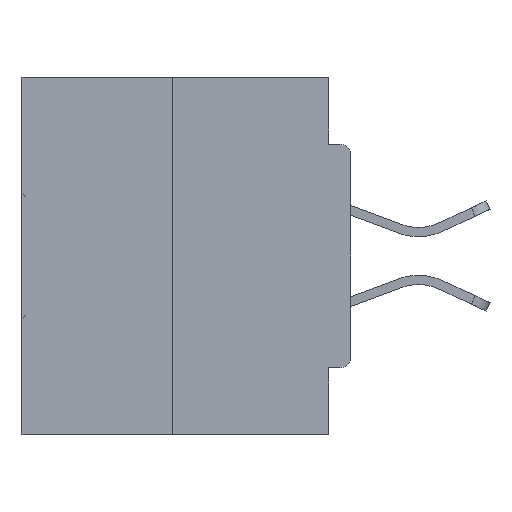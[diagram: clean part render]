
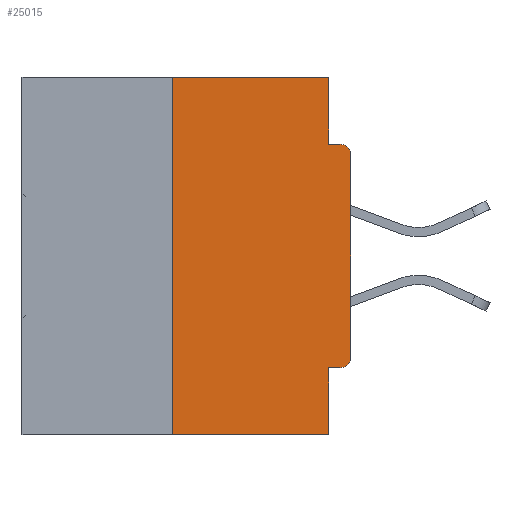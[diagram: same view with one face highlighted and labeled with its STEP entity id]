
A CAD part, left-side view. The second image highlights one B-rep face of the part: STEP entity #25015.
In plain terms, the highlighted planar face has unit normal (-1, 0, 0).
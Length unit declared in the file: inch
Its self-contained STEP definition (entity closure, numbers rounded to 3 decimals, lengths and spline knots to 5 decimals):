
#209 = VERTEX_POINT ( 'NONE', #27853 ) ;
#298 = CARTESIAN_POINT ( 'NONE',  ( 0., 0.25, 0. ) ) ;
#849 = ORIENTED_EDGE ( 'NONE', *, *, #33226, .T. ) ;
#915 = VECTOR ( 'NONE', #22588, 39.37008 ) ;
#1058 = LINE ( 'NONE', #39771, #12234 ) ;
#1157 = DIRECTION ( 'NONE',  ( 0., 0., -1. ) ) ;
#1381 = CARTESIAN_POINT ( 'NONE',  ( 0., 0., -0.4065 ) ) ;
#1384 = VERTEX_POINT ( 'NONE', #38906 ) ;
#1772 = ORIENTED_EDGE ( 'NONE', *, *, #12917, .T. ) ;
#2313 = CARTESIAN_POINT ( 'NONE',  ( 0., 0.031, -0.5 ) ) ;
#2521 = ORIENTED_EDGE ( 'NONE', *, *, #5078, .T. ) ;
#3207 = CARTESIAN_POINT ( 'NONE',  ( 0., 0.031, -0.4065 ) ) ;
#3614 = EDGE_CURVE ( 'NONE', #1384, #21017, #34693, .T. ) ;
#3821 = LINE ( 'NONE', #11021, #28789 ) ;
#3996 = VERTEX_POINT ( 'NONE', #16469 ) ;
#5057 = ORIENTED_EDGE ( 'NONE', *, *, #3614, .F. ) ;
#5078 = EDGE_CURVE ( 'NONE', #3996, #27350, #22658, .T. ) ;
#5991 = EDGE_CURVE ( 'NONE', #209, #16376, #36353, .T. ) ;
#6490 = CARTESIAN_POINT ( 'NONE',  ( 0., 0.25, 0. ) ) ;
#6495 = LINE ( 'NONE', #22873, #915 ) ;
#8624 = EDGE_CURVE ( 'NONE', #27197, #25356, #6495, .T. ) ;
#9118 = CARTESIAN_POINT ( 'NONE',  ( 0., 0.015, -0.3915 ) ) ;
#9577 = CARTESIAN_POINT ( 'NONE',  ( 0., 0., 0. ) ) ;
#10607 = VERTEX_POINT ( 'NONE', #32449 ) ;
#10872 = CARTESIAN_POINT ( 'NONE',  ( 0., 0.031, -0.5 ) ) ;
#11021 = CARTESIAN_POINT ( 'NONE',  ( 0., 0.46, -0.5 ) ) ;
#11678 = EDGE_LOOP ( 'NONE', ( #41995, #12970, #14958, #31051, #5057, #1772, #2521, #849, #37008, #13912 ) ) ;
#11947 = DIRECTION ( 'NONE',  ( 0., -1., 0. ) ) ;
#12234 = VECTOR ( 'NONE', #40074, 39.37008 ) ;
#12376 = DIRECTION ( 'NONE',  ( 0., 0., -1. ) ) ;
#12406 = DIRECTION ( 'NONE',  ( 0., 0., 1. ) ) ;
#12452 = VECTOR ( 'NONE', #11947, 39.37008 ) ;
#12458 = EDGE_CURVE ( 'NONE', #25356, #10607, #29871, .T. ) ;
#12851 = VERTEX_POINT ( 'NONE', #10872 ) ;
#12860 = EDGE_CURVE ( 'NONE', #209, #12851, #3821, .T. ) ;
#12917 = EDGE_CURVE ( 'NONE', #1384, #3996, #36448, .T. ) ;
#12970 = ORIENTED_EDGE ( 'NONE', *, *, #5991, .F. ) ;
#13542 = LINE ( 'NONE', #2313, #17114 ) ;
#13912 = ORIENTED_EDGE ( 'NONE', *, *, #8624, .F. ) ;
#14000 = DIRECTION ( 'NONE',  ( -1., 0., 0. ) ) ;
#14783 = DIRECTION ( 'NONE',  ( 1., 0., 0. ) ) ;
#14942 = CIRCLE ( 'NONE', #29311, 0.015 ) ;
#14958 = ORIENTED_EDGE ( 'NONE', *, *, #12860, .T. ) ;
#15092 = CARTESIAN_POINT ( 'NONE',  ( 0., 0.031, 0. ) ) ;
#15818 = FACE_OUTER_BOUND ( 'NONE', #11678, .T. ) ;
#16376 = VERTEX_POINT ( 'NONE', #6490 ) ;
#16469 = CARTESIAN_POINT ( 'NONE',  ( 0., 0., -0.3915 ) ) ;
#17087 = VECTOR ( 'NONE', #12406, 39.37008 ) ;
#17114 = VECTOR ( 'NONE', #29705, 39.37008 ) ;
#18168 = CARTESIAN_POINT ( 'NONE',  ( 0., 0.031, -0.0935 ) ) ;
#19508 = VECTOR ( 'NONE', #33560, 39.37008 ) ;
#19795 = AXIS2_PLACEMENT_3D ( 'NONE', #34484, #14783, #37616 ) ;
#21017 = VERTEX_POINT ( 'NONE', #3207 ) ;
#22588 = DIRECTION ( 'NONE',  ( 0., 0., -1. ) ) ;
#22658 = LINE ( 'NONE', #9577, #17087 ) ;
#22873 = CARTESIAN_POINT ( 'NONE',  ( 0., 0.031, 0. ) ) ;
#25015 = ADVANCED_FACE ( 'NONE', ( #15818 ), #34359, .F. ) ;
#25356 = VERTEX_POINT ( 'NONE', #18168 ) ;
#26029 = VECTOR ( 'NONE', #37715, 39.37008 ) ;
#26883 = DIRECTION ( 'NONE',  ( 0., -1., 0. ) ) ;
#27197 = VERTEX_POINT ( 'NONE', #15092 ) ;
#27350 = VERTEX_POINT ( 'NONE', #38610 ) ;
#27853 = CARTESIAN_POINT ( 'NONE',  ( 0., 0.25, -0.5 ) ) ;
#28789 = VECTOR ( 'NONE', #26883, 39.37008 ) ;
#28820 = EDGE_CURVE ( 'NONE', #21017, #12851, #13542, .T. ) ;
#29311 = AXIS2_PLACEMENT_3D ( 'NONE', #40356, #14000, #1157 ) ;
#29705 = DIRECTION ( 'NONE',  ( 0., 0., -1. ) ) ;
#29871 = LINE ( 'NONE', #38455, #12452 ) ;
#29897 = AXIS2_PLACEMENT_3D ( 'NONE', #9118, #31951, #12376 ) ;
#31051 = ORIENTED_EDGE ( 'NONE', *, *, #28820, .F. ) ;
#31951 = DIRECTION ( 'NONE',  ( -1., 0., 0. ) ) ;
#32449 = CARTESIAN_POINT ( 'NONE',  ( 0., 0.015, -0.0935 ) ) ;
#33226 = EDGE_CURVE ( 'NONE', #27350, #10607, #14942, .T. ) ;
#33560 = DIRECTION ( 'NONE',  ( 0., 0., 1. ) ) ;
#34359 = PLANE ( 'NONE',  #19795 ) ;
#34484 = CARTESIAN_POINT ( 'NONE',  ( 0., 0.46, 0. ) ) ;
#34488 = EDGE_CURVE ( 'NONE', #16376, #27197, #1058, .T. ) ;
#34693 = LINE ( 'NONE', #1381, #26029 ) ;
#36353 = LINE ( 'NONE', #298, #19508 ) ;
#36448 = CIRCLE ( 'NONE', #29897, 0.015 ) ;
#37008 = ORIENTED_EDGE ( 'NONE', *, *, #12458, .F. ) ;
#37616 = DIRECTION ( 'NONE',  ( 0., 0., -1. ) ) ;
#37715 = DIRECTION ( 'NONE',  ( 0., 1., 0. ) ) ;
#38455 = CARTESIAN_POINT ( 'NONE',  ( 0., 0., -0.0935 ) ) ;
#38610 = CARTESIAN_POINT ( 'NONE',  ( 0., 0., -0.1085 ) ) ;
#38906 = CARTESIAN_POINT ( 'NONE',  ( 0., 0.015, -0.4065 ) ) ;
#39771 = CARTESIAN_POINT ( 'NONE',  ( 0., 0.46, 0. ) ) ;
#40074 = DIRECTION ( 'NONE',  ( 0., -1., 0. ) ) ;
#40356 = CARTESIAN_POINT ( 'NONE',  ( 0., 0.015, -0.1085 ) ) ;
#41995 = ORIENTED_EDGE ( 'NONE', *, *, #34488, .F. ) ;
